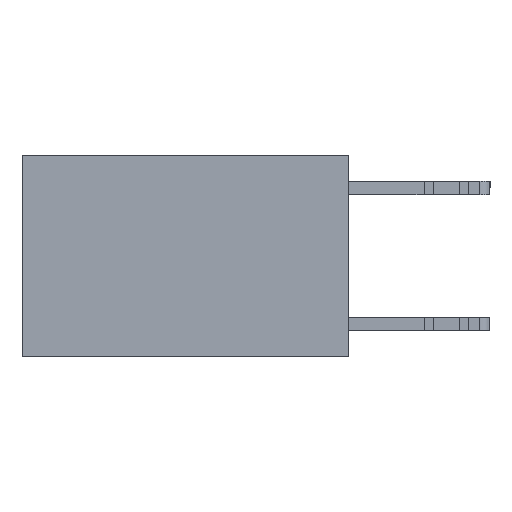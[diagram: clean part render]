
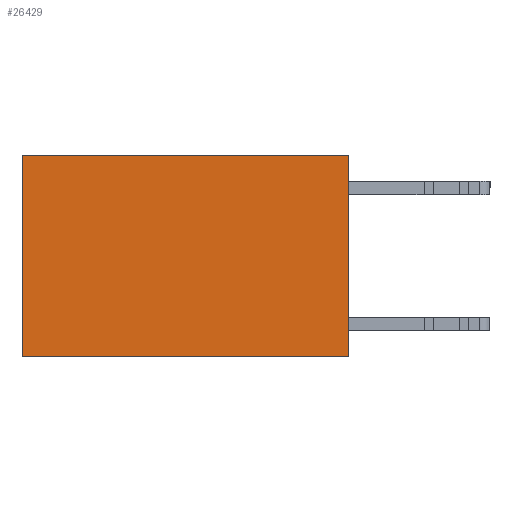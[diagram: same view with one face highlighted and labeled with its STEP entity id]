
A CAD part, left-side view. The second image highlights one B-rep face of the part: STEP entity #26429.
In plain terms, the highlighted planar face has unit normal (-1, 0, 0).
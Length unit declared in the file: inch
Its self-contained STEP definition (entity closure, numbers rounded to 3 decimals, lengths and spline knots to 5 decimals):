
#1207 = FACE_OUTER_BOUND ( 'NONE', #9921, .T. ) ;
#2236 = DIRECTION ( 'NONE',  ( 0., 0., -1. ) ) ;
#4478 = VERTEX_POINT ( 'NONE', #17672 ) ;
#6538 = LINE ( 'NONE', #24769, #21625 ) ;
#7624 = EDGE_CURVE ( 'NONE', #9724, #4478, #22654, .T. ) ;
#9532 = ORIENTED_EDGE ( 'NONE', *, *, #18946, .T. ) ;
#9724 = VERTEX_POINT ( 'NONE', #10311 ) ;
#9821 = CARTESIAN_POINT ( 'NONE',  ( 0.2625, 0.6, -0.37 ) ) ;
#9921 = EDGE_LOOP ( 'NONE', ( #9532, #25855, #19085, #29616 ) ) ;
#10311 = CARTESIAN_POINT ( 'NONE',  ( 0.2625, 0., 0. ) ) ;
#10563 = CARTESIAN_POINT ( 'NONE',  ( 0.2625, 0., 0. ) ) ;
#11400 = VERTEX_POINT ( 'NONE', #9821 ) ;
#13973 = VECTOR ( 'NONE', #28041, 39.37008 ) ;
#14429 = CARTESIAN_POINT ( 'NONE',  ( 0.2625, 0., 0. ) ) ;
#15085 = VECTOR ( 'NONE', #25573, 39.37008 ) ;
#16255 = LINE ( 'NONE', #23565, #15085 ) ;
#16275 = LINE ( 'NONE', #14429, #13973 ) ;
#16630 = EDGE_CURVE ( 'NONE', #26038, #11400, #16255, .T. ) ;
#17631 = AXIS2_PLACEMENT_3D ( 'NONE', #10563, #19916, #29224 ) ;
#17672 = CARTESIAN_POINT ( 'NONE',  ( 0.2625, 0.6, 0. ) ) ;
#18946 = EDGE_CURVE ( 'NONE', #4478, #11400, #6538, .T. ) ;
#19085 = ORIENTED_EDGE ( 'NONE', *, *, #23318, .F. ) ;
#19916 = DIRECTION ( 'NONE',  ( 1., 0., 0. ) ) ;
#20371 = CARTESIAN_POINT ( 'NONE',  ( 0.2625, 0., 0. ) ) ;
#21606 = VECTOR ( 'NONE', #22503, 39.37008 ) ;
#21625 = VECTOR ( 'NONE', #2236, 39.37008 ) ;
#22503 = DIRECTION ( 'NONE',  ( 0., 1., 0. ) ) ;
#22654 = LINE ( 'NONE', #20371, #21606 ) ;
#23318 = EDGE_CURVE ( 'NONE', #9724, #26038, #16275, .T. ) ;
#23565 = CARTESIAN_POINT ( 'NONE',  ( 0.2625, 0., -0.37 ) ) ;
#24769 = CARTESIAN_POINT ( 'NONE',  ( 0.2625, 0.6, 0. ) ) ;
#25573 = DIRECTION ( 'NONE',  ( 0., 1., 0. ) ) ;
#25855 = ORIENTED_EDGE ( 'NONE', *, *, #16630, .F. ) ;
#26038 = VERTEX_POINT ( 'NONE', #29702 ) ;
#26429 = ADVANCED_FACE ( 'NONE', ( #1207 ), #26937, .F. ) ;
#26937 = PLANE ( 'NONE',  #17631 ) ;
#28041 = DIRECTION ( 'NONE',  ( 0., 0., -1. ) ) ;
#29224 = DIRECTION ( 'NONE',  ( 0., 0., -1. ) ) ;
#29616 = ORIENTED_EDGE ( 'NONE', *, *, #7624, .T. ) ;
#29702 = CARTESIAN_POINT ( 'NONE',  ( 0.2625, 0., -0.37 ) ) ;
